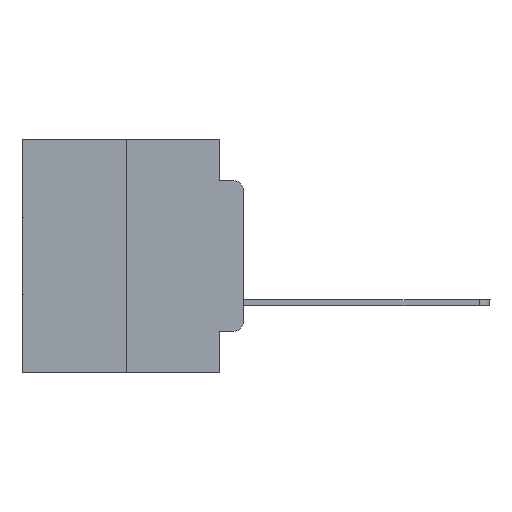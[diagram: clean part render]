
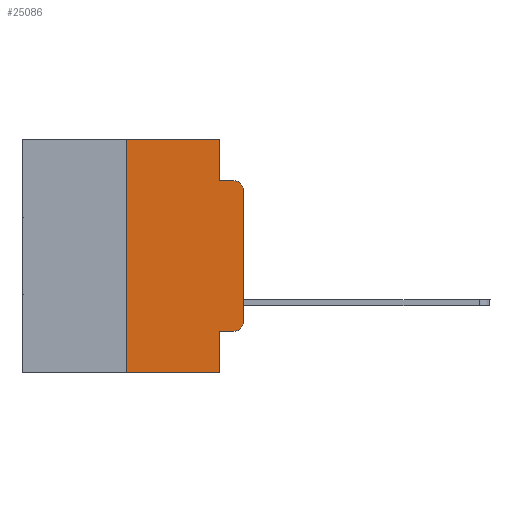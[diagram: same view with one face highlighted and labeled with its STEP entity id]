
A CAD part, left-side view. The second image highlights one B-rep face of the part: STEP entity #25086.
In plain terms, the highlighted planar face has unit normal (-1, 0, 0).
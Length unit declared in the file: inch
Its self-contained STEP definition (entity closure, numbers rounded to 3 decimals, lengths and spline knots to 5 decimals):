
#224 = DIRECTION ( 'NONE',  ( 0., -1., 0. ) ) ;
#505 = DIRECTION ( 'NONE',  ( 0., 0., -1. ) ) ;
#823 = EDGE_LOOP ( 'NONE', ( #21367, #27836, #16362, #29027, #26276, #13566, #20601, #9202, #13477, #18014 ) ) ;
#1321 = DIRECTION ( 'NONE',  ( 0., 0., -1. ) ) ;
#1428 = AXIS2_PLACEMENT_3D ( 'NONE', #21719, #19214, #1321 ) ;
#1682 = CARTESIAN_POINT ( 'NONE',  ( 0., 0.02, -0.0885 ) ) ;
#2104 = CARTESIAN_POINT ( 'NONE',  ( 0., 0.25, -0.5 ) ) ;
#2452 = LINE ( 'NONE', #21291, #8103 ) ;
#2505 = VERTEX_POINT ( 'NONE', #4083 ) ;
#2803 = VERTEX_POINT ( 'NONE', #26157 ) ;
#3508 = LINE ( 'NONE', #8187, #11974 ) ;
#3671 = LINE ( 'NONE', #27618, #8992 ) ;
#4083 = CARTESIAN_POINT ( 'NONE',  ( 0., 0.25, 0. ) ) ;
#4814 = LINE ( 'NONE', #21192, #21129 ) ;
#4830 = VECTOR ( 'NONE', #224, 39.37008 ) ;
#5221 = CARTESIAN_POINT ( 'NONE',  ( 0., 0.473, 0. ) ) ;
#5762 = VERTEX_POINT ( 'NONE', #25700 ) ;
#5803 = EDGE_CURVE ( 'NONE', #9348, #2803, #20429, .T. ) ;
#5818 = CIRCLE ( 'NONE', #28640, 0.02 ) ;
#8103 = VECTOR ( 'NONE', #25861, 39.37008 ) ;
#8187 = CARTESIAN_POINT ( 'NONE',  ( 0., 0., 0. ) ) ;
#8386 = VECTOR ( 'NONE', #27860, 39.37008 ) ;
#8414 = CARTESIAN_POINT ( 'NONE',  ( 0., 0.051, 0. ) ) ;
#8610 = EDGE_CURVE ( 'NONE', #21945, #21700, #2452, .T. ) ;
#8991 = VERTEX_POINT ( 'NONE', #12344 ) ;
#8992 = VECTOR ( 'NONE', #505, 39.37008 ) ;
#9091 = EDGE_CURVE ( 'NONE', #5762, #9455, #3508, .T. ) ;
#9202 = ORIENTED_EDGE ( 'NONE', *, *, #11590, .F. ) ;
#9348 = VERTEX_POINT ( 'NONE', #2104 ) ;
#9455 = VERTEX_POINT ( 'NONE', #15179 ) ;
#9747 = CARTESIAN_POINT ( 'NONE',  ( 0., 0.051, -0.4115 ) ) ;
#10754 = VERTEX_POINT ( 'NONE', #9747 ) ;
#10830 = VECTOR ( 'NONE', #21296, 39.37008 ) ;
#10990 = EDGE_CURVE ( 'NONE', #9348, #2505, #4814, .T. ) ;
#11040 = EDGE_CURVE ( 'NONE', #2505, #16924, #20728, .T. ) ;
#11100 = DIRECTION ( 'NONE',  ( -1., 0., 0. ) ) ;
#11301 = DIRECTION ( 'NONE',  ( 1., 0., 0. ) ) ;
#11590 = EDGE_CURVE ( 'NONE', #10754, #2803, #23563, .T. ) ;
#11974 = VECTOR ( 'NONE', #15246, 39.37008 ) ;
#12185 = DIRECTION ( 'NONE',  ( 0., 0., 1. ) ) ;
#12344 = CARTESIAN_POINT ( 'NONE',  ( 0., 0.02, -0.4115 ) ) ;
#12661 = EDGE_CURVE ( 'NONE', #16924, #21945, #3671, .T. ) ;
#13477 = ORIENTED_EDGE ( 'NONE', *, *, #16126, .T. ) ;
#13489 = DIRECTION ( 'NONE',  ( 0., 0., -1. ) ) ;
#13566 = ORIENTED_EDGE ( 'NONE', *, *, #10990, .F. ) ;
#13793 = CARTESIAN_POINT ( 'NONE',  ( 0., 0.051, -0.4115 ) ) ;
#14336 = CARTESIAN_POINT ( 'NONE',  ( 0., 0.051, 0. ) ) ;
#15179 = CARTESIAN_POINT ( 'NONE',  ( 0., 0., -0.1085 ) ) ;
#15246 = DIRECTION ( 'NONE',  ( 0., 0., 1. ) ) ;
#16064 = CARTESIAN_POINT ( 'NONE',  ( 0., 0.473, 0. ) ) ;
#16126 = EDGE_CURVE ( 'NONE', #10754, #8991, #17608, .T. ) ;
#16362 = ORIENTED_EDGE ( 'NONE', *, *, #8610, .F. ) ;
#16487 = VECTOR ( 'NONE', #23747, 39.37008 ) ;
#16840 = EDGE_CURVE ( 'NONE', #8991, #5762, #5818, .T. ) ;
#16924 = VERTEX_POINT ( 'NONE', #8414 ) ;
#17608 = LINE ( 'NONE', #13793, #4830 ) ;
#18014 = ORIENTED_EDGE ( 'NONE', *, *, #16840, .T. ) ;
#19214 = DIRECTION ( 'NONE',  ( -1., 0., 0. ) ) ;
#20003 = CARTESIAN_POINT ( 'NONE',  ( 0., 0.02, -0.3915 ) ) ;
#20429 = LINE ( 'NONE', #23037, #8386 ) ;
#20601 = ORIENTED_EDGE ( 'NONE', *, *, #5803, .T. ) ;
#20683 = PLANE ( 'NONE',  #26732 ) ;
#20728 = LINE ( 'NONE', #5221, #10830 ) ;
#20815 = FACE_OUTER_BOUND ( 'NONE', #823, .T. ) ;
#21082 = EDGE_CURVE ( 'NONE', #9455, #21700, #26190, .T. ) ;
#21129 = VECTOR ( 'NONE', #12185, 39.37008 ) ;
#21192 = CARTESIAN_POINT ( 'NONE',  ( 0., 0.25, 0. ) ) ;
#21291 = CARTESIAN_POINT ( 'NONE',  ( 0., 0.051, -0.0885 ) ) ;
#21296 = DIRECTION ( 'NONE',  ( 0., -1., 0. ) ) ;
#21367 = ORIENTED_EDGE ( 'NONE', *, *, #9091, .T. ) ;
#21700 = VERTEX_POINT ( 'NONE', #1682 ) ;
#21719 = CARTESIAN_POINT ( 'NONE',  ( 0., 0.02, -0.1085 ) ) ;
#21945 = VERTEX_POINT ( 'NONE', #22578 ) ;
#22578 = CARTESIAN_POINT ( 'NONE',  ( 0., 0.051, -0.0885 ) ) ;
#23037 = CARTESIAN_POINT ( 'NONE',  ( 0., 0.473, -0.5 ) ) ;
#23563 = LINE ( 'NONE', #14336, #16487 ) ;
#23747 = DIRECTION ( 'NONE',  ( 0., 0., -1. ) ) ;
#25086 = ADVANCED_FACE ( 'NONE', ( #20815 ), #20683, .F. ) ;
#25700 = CARTESIAN_POINT ( 'NONE',  ( 0., 0., -0.3915 ) ) ;
#25861 = DIRECTION ( 'NONE',  ( 0., -1., 0. ) ) ;
#26157 = CARTESIAN_POINT ( 'NONE',  ( 0., 0.051, -0.5 ) ) ;
#26190 = CIRCLE ( 'NONE', #1428, 0.02 ) ;
#26276 = ORIENTED_EDGE ( 'NONE', *, *, #11040, .F. ) ;
#26732 = AXIS2_PLACEMENT_3D ( 'NONE', #16064, #11301, #13489 ) ;
#27618 = CARTESIAN_POINT ( 'NONE',  ( 0., 0.051, 0. ) ) ;
#27836 = ORIENTED_EDGE ( 'NONE', *, *, #21082, .T. ) ;
#27860 = DIRECTION ( 'NONE',  ( 0., -1., 0. ) ) ;
#28640 = AXIS2_PLACEMENT_3D ( 'NONE', #20003, #11100, #28926 ) ;
#28926 = DIRECTION ( 'NONE',  ( 0., 0., -1. ) ) ;
#29027 = ORIENTED_EDGE ( 'NONE', *, *, #12661, .F. ) ;
